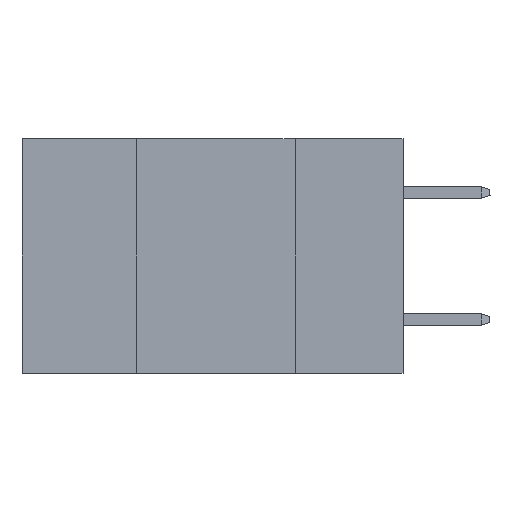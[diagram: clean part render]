
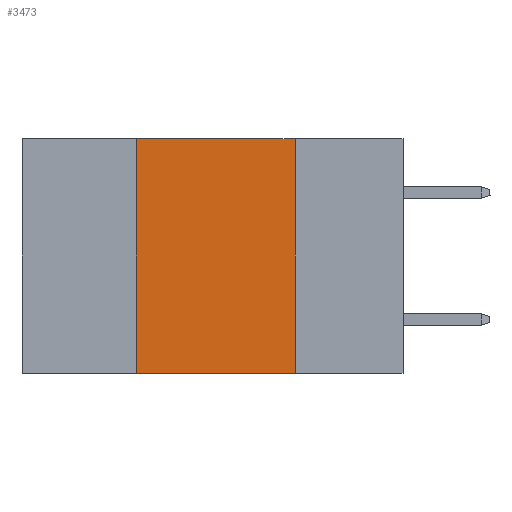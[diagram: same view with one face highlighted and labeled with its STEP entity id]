
A CAD part, left-side view. The second image highlights one B-rep face of the part: STEP entity #3473.
In plain terms, the highlighted planar face has unit normal (-1, 0, 0).
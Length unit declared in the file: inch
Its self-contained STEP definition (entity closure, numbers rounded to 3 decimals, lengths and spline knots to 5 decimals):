
#105 = DIRECTION ( 'NONE',  ( 0., 0., 1. ) ) ;
#1143 = DIRECTION ( 'NONE',  ( 1., 0., 0. ) ) ;
#1608 = CARTESIAN_POINT ( 'NONE',  ( 0., 0.6, -0.37 ) ) ;
#2029 = LINE ( 'NONE', #14073, #15062 ) ;
#2586 = VERTEX_POINT ( 'NONE', #14828 ) ;
#2639 = DIRECTION ( 'NONE',  ( 0., 0., -1. ) ) ;
#2653 = DIRECTION ( 'NONE',  ( 0., 0., -1. ) ) ;
#2692 = EDGE_CURVE ( 'NONE', #21675, #14810, #19628, .T. ) ;
#3128 = VECTOR ( 'NONE', #2653, 39.37008 ) ;
#3473 = ADVANCED_FACE ( 'NONE', ( #16854 ), #11341, .F. ) ;
#3960 = ORIENTED_EDGE ( 'NONE', *, *, #2692, .T. ) ;
#4204 = VERTEX_POINT ( 'NONE', #5873 ) ;
#4313 = LINE ( 'NONE', #7897, #14967 ) ;
#4561 = CARTESIAN_POINT ( 'NONE',  ( 0., 0.6, 0. ) ) ;
#5873 = CARTESIAN_POINT ( 'NONE',  ( 0., 0.42, 0. ) ) ;
#5939 = AXIS2_PLACEMENT_3D ( 'NONE', #4561, #1143, #2639 ) ;
#5966 = ORIENTED_EDGE ( 'NONE', *, *, #6469, .F. ) ;
#6469 = EDGE_CURVE ( 'NONE', #21675, #4204, #2029, .T. ) ;
#7897 = CARTESIAN_POINT ( 'NONE',  ( 0., 0.6, 0. ) ) ;
#8499 = ORIENTED_EDGE ( 'NONE', *, *, #13816, .F. ) ;
#9005 = CARTESIAN_POINT ( 'NONE',  ( 0., 0.42, -0.37 ) ) ;
#11341 = PLANE ( 'NONE',  #5939 ) ;
#12965 = LINE ( 'NONE', #18386, #3128 ) ;
#13159 = CARTESIAN_POINT ( 'NONE',  ( 0., 0.17, -0.37 ) ) ;
#13816 = EDGE_CURVE ( 'NONE', #2586, #14810, #12965, .T. ) ;
#13988 = DIRECTION ( 'NONE',  ( 0., -1., 0. ) ) ;
#14073 = CARTESIAN_POINT ( 'NONE',  ( 0., 0.42, 0. ) ) ;
#14171 = VECTOR ( 'NONE', #13988, 39.37008 ) ;
#14810 = VERTEX_POINT ( 'NONE', #13159 ) ;
#14828 = CARTESIAN_POINT ( 'NONE',  ( 0., 0.17, 0. ) ) ;
#14967 = VECTOR ( 'NONE', #20092, 39.37008 ) ;
#15062 = VECTOR ( 'NONE', #105, 39.37008 ) ;
#15115 = EDGE_LOOP ( 'NONE', ( #8499, #21768, #5966, #3960 ) ) ;
#16854 = FACE_OUTER_BOUND ( 'NONE', #15115, .T. ) ;
#18386 = CARTESIAN_POINT ( 'NONE',  ( 0., 0.17, 0. ) ) ;
#19628 = LINE ( 'NONE', #1608, #14171 ) ;
#20092 = DIRECTION ( 'NONE',  ( 0., -1., 0. ) ) ;
#21675 = VERTEX_POINT ( 'NONE', #9005 ) ;
#21768 = ORIENTED_EDGE ( 'NONE', *, *, #22395, .F. ) ;
#22395 = EDGE_CURVE ( 'NONE', #4204, #2586, #4313, .T. ) ;
